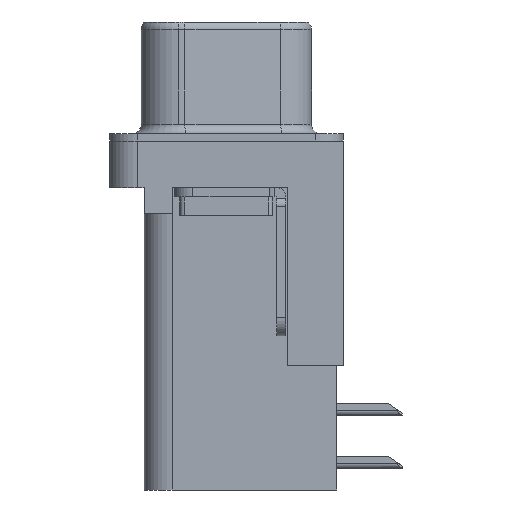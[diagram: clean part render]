
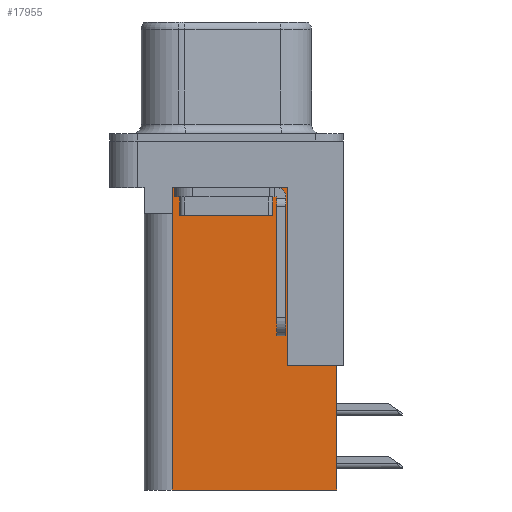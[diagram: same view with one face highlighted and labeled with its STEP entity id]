
A CAD part, left-side view. The second image highlights one B-rep face of the part: STEP entity #17955.
In plain terms, the highlighted planar face has unit normal (-1, 0, 0).
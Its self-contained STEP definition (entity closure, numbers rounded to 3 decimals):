
#1248 = ORIENTED_EDGE ( 'NONE', *, *, #12300, .T. ) ;
#1436 = CARTESIAN_POINT ( 'NONE',  ( 3.765, -5.925, -12.05 ) ) ;
#1502 = ORIENTED_EDGE ( 'NONE', *, *, #16895, .T. ) ;
#1880 = DIRECTION ( 'NONE',  ( 1., 0., 0. ) ) ;
#2037 = DIRECTION ( 'NONE',  ( 0., 0., -1. ) ) ;
#2187 = VECTOR ( 'NONE', #15224, 1000. ) ;
#2291 = CARTESIAN_POINT ( 'NONE',  ( 3.765, 2.895, -3.9 ) ) ;
#3117 = VECTOR ( 'NONE', #17548, 1000. ) ;
#3366 = CARTESIAN_POINT ( 'NONE',  ( 3.765, -3.295, -18.76 ) ) ;
#3463 = CARTESIAN_POINT ( 'NONE',  ( 3.765, -5.925, -2. ) ) ;
#3663 = DIRECTION ( 'NONE',  ( 0., 1., 0. ) ) ;
#4119 = DIRECTION ( 'NONE',  ( 0., 1., 0. ) ) ;
#4341 = CARTESIAN_POINT ( 'NONE',  ( 3.765, 2.925, -18.76 ) ) ;
#4407 = CARTESIAN_POINT ( 'NONE',  ( 3.765, -3.295, -18.76 ) ) ;
#4573 = VERTEX_POINT ( 'NONE', #4341 ) ;
#4616 = VECTOR ( 'NONE', #3663, 1000. ) ;
#4691 = VERTEX_POINT ( 'NONE', #9113 ) ;
#5692 = EDGE_CURVE ( 'NONE', #10138, #4691, #13334, .T. ) ;
#5732 = ORIENTED_EDGE ( 'NONE', *, *, #10623, .T. ) ;
#6220 = LINE ( 'NONE', #3463, #2187 ) ;
#6639 = LINE ( 'NONE', #7364, #3117 ) ;
#6907 = VECTOR ( 'NONE', #13697, 1000. ) ;
#7364 = CARTESIAN_POINT ( 'NONE',  ( 3.765, 2.925, -18.76 ) ) ;
#8150 = CARTESIAN_POINT ( 'NONE',  ( 3.765, -3.295, -12.05 ) ) ;
#8223 = EDGE_LOOP ( 'NONE', ( #5732, #17707, #1248, #14528, #17669, #10299, #1502, #16753 ) ) ;
#8558 = LINE ( 'NONE', #9584, #4616 ) ;
#8841 = CARTESIAN_POINT ( 'NONE',  ( 3.765, 0., -3.9 ) ) ;
#9113 = CARTESIAN_POINT ( 'NONE',  ( 3.765, 2.895, -3.9 ) ) ;
#9392 = CARTESIAN_POINT ( 'NONE',  ( 3.765, -5.925, -18.76 ) ) ;
#9584 = CARTESIAN_POINT ( 'NONE',  ( 3.765, -3.295, -2.5 ) ) ;
#9743 = VERTEX_POINT ( 'NONE', #13848 ) ;
#9794 = CARTESIAN_POINT ( 'NONE',  ( 3.765, 2.925, -3.9 ) ) ;
#9911 = LINE ( 'NONE', #14381, #14188 ) ;
#10138 = VERTEX_POINT ( 'NONE', #19022 ) ;
#10299 = ORIENTED_EDGE ( 'NONE', *, *, #16595, .F. ) ;
#10537 = VERTEX_POINT ( 'NONE', #9392 ) ;
#10623 = EDGE_CURVE ( 'NONE', #9743, #10138, #8558, .T. ) ;
#10788 = PLANE ( 'NONE',  #16273 ) ;
#10821 = LINE ( 'NONE', #4407, #11738 ) ;
#11240 = LINE ( 'NONE', #8841, #14632 ) ;
#11433 = FACE_OUTER_BOUND ( 'NONE', #8223, .T. ) ;
#11738 = VECTOR ( 'NONE', #14639, 1000. ) ;
#12252 = DIRECTION ( 'NONE',  ( 0., 1., 0. ) ) ;
#12300 = EDGE_CURVE ( 'NONE', #4691, #14154, #11240, .T. ) ;
#13334 = LINE ( 'NONE', #2291, #17238 ) ;
#13697 = DIRECTION ( 'NONE',  ( 0., 1., 0. ) ) ;
#13848 = CARTESIAN_POINT ( 'NONE',  ( 3.765, -3.295, -2.5 ) ) ;
#14154 = VERTEX_POINT ( 'NONE', #9794 ) ;
#14188 = VECTOR ( 'NONE', #4119, 1000. ) ;
#14381 = CARTESIAN_POINT ( 'NONE',  ( 3.765, -6.295, -12.05 ) ) ;
#14528 = ORIENTED_EDGE ( 'NONE', *, *, #18900, .F. ) ;
#14623 = LINE ( 'NONE', #3366, #6907 ) ;
#14632 = VECTOR ( 'NONE', #17555, 1000. ) ;
#14639 = DIRECTION ( 'NONE',  ( 0., 0., 1. ) ) ;
#15224 = DIRECTION ( 'NONE',  ( 0., 0., -1. ) ) ;
#16273 = AXIS2_PLACEMENT_3D ( 'NONE', #16622, #1880, #12252 ) ;
#16309 = EDGE_CURVE ( 'NONE', #16693, #9743, #10821, .T. ) ;
#16595 = EDGE_CURVE ( 'NONE', #17714, #10537, #6220, .T. ) ;
#16622 = CARTESIAN_POINT ( 'NONE',  ( 3.765, -3.295, -18.76 ) ) ;
#16693 = VERTEX_POINT ( 'NONE', #8150 ) ;
#16753 = ORIENTED_EDGE ( 'NONE', *, *, #16309, .T. ) ;
#16895 = EDGE_CURVE ( 'NONE', #17714, #16693, #9911, .T. ) ;
#17238 = VECTOR ( 'NONE', #2037, 1000. ) ;
#17258 = EDGE_CURVE ( 'NONE', #10537, #4573, #14623, .T. ) ;
#17548 = DIRECTION ( 'NONE',  ( 0., 0., 1. ) ) ;
#17555 = DIRECTION ( 'NONE',  ( 0., 1., 0. ) ) ;
#17669 = ORIENTED_EDGE ( 'NONE', *, *, #17258, .F. ) ;
#17707 = ORIENTED_EDGE ( 'NONE', *, *, #5692, .T. ) ;
#17714 = VERTEX_POINT ( 'NONE', #1436 ) ;
#17955 = ADVANCED_FACE ( 'NONE', ( #11433 ), #10788, .F. ) ;
#18900 = EDGE_CURVE ( 'NONE', #4573, #14154, #6639, .T. ) ;
#19022 = CARTESIAN_POINT ( 'NONE',  ( 3.765, 2.895, -2.5 ) ) ;
